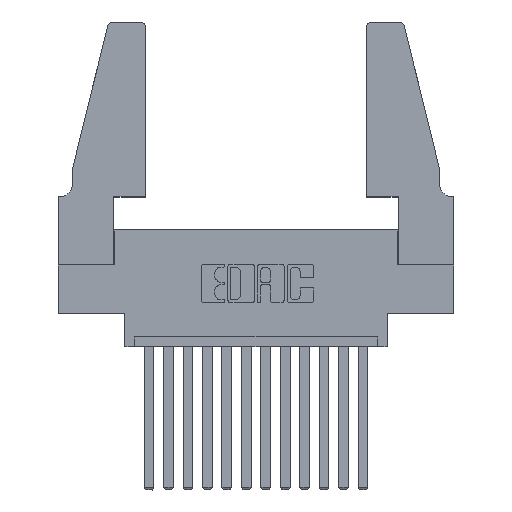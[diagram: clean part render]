
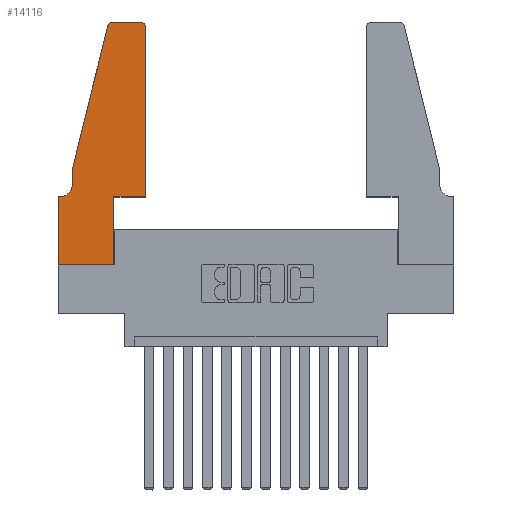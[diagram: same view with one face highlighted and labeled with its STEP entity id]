
A CAD part, top view. The second image highlights one B-rep face of the part: STEP entity #14116.
In plain terms, the highlighted planar face has unit normal (0, 0, 1).
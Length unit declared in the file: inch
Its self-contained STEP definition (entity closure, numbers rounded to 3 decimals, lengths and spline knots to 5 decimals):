
#272 = LINE ( 'NONE', #6849, #1726 ) ;
#416 = DIRECTION ( 'NONE',  ( 0., 0., 1. ) ) ;
#508 = EDGE_CURVE ( 'NONE', #1469, #7959, #272, .T. ) ;
#634 = DIRECTION ( 'NONE',  ( 0., 0., 1. ) ) ;
#906 = CARTESIAN_POINT ( 'NONE',  ( 0.0055, 0.35, 0.37 ) ) ;
#988 = LINE ( 'NONE', #8425, #2473 ) ;
#1020 = CARTESIAN_POINT ( 'NONE',  ( 0., 0.35, 0.37 ) ) ;
#1269 = DIRECTION ( 'NONE',  ( 0., -1., 0. ) ) ;
#1311 = CARTESIAN_POINT ( 'NONE',  ( 0.2865, 0.35, 0.37 ) ) ;
#1469 = VERTEX_POINT ( 'NONE', #1020 ) ;
#1584 = EDGE_CURVE ( 'NONE', #9518, #4187, #13650, .T. ) ;
#1589 = VERTEX_POINT ( 'NONE', #7172 ) ;
#1726 = VECTOR ( 'NONE', #7943, 39.37008 ) ;
#1871 = CARTESIAN_POINT ( 'NONE',  ( 0.4505, 0.35, 0.37 ) ) ;
#2280 = CARTESIAN_POINT ( 'NONE',  ( 0.4205, 1.25, 0.37 ) ) ;
#2445 = CARTESIAN_POINT ( 'NONE',  ( 0.284, 1.25, 0.37 ) ) ;
#2473 = VECTOR ( 'NONE', #1269, 39.37008 ) ;
#2568 = CARTESIAN_POINT ( 'NONE',  ( 0.4205, 1.22, 0.37 ) ) ;
#2576 = DIRECTION ( 'NONE',  ( 1., 0., 0. ) ) ;
#2619 = AXIS2_PLACEMENT_3D ( 'NONE', #14157, #12013, #7333 ) ;
#2770 = CARTESIAN_POINT ( 'NONE',  ( 0., 0., 0.37 ) ) ;
#3137 = EDGE_CURVE ( 'NONE', #7294, #11831, #12317, .T. ) ;
#3574 = EDGE_CURVE ( 'NONE', #11831, #5307, #11394, .T. ) ;
#3768 = VECTOR ( 'NONE', #7999, 39.37008 ) ;
#3900 = DIRECTION ( 'NONE',  ( 1., 0., 0. ) ) ;
#4038 = PLANE ( 'NONE',  #8104 ) ;
#4187 = VERTEX_POINT ( 'NONE', #906 ) ;
#4556 = EDGE_CURVE ( 'NONE', #4187, #1469, #12631, .T. ) ;
#4632 = FACE_OUTER_BOUND ( 'NONE', #12055, .T. ) ;
#4731 = VERTEX_POINT ( 'NONE', #11976 ) ;
#5307 = VERTEX_POINT ( 'NONE', #2445 ) ;
#5340 = DIRECTION ( 'NONE',  ( 0., 1., 0. ) ) ;
#5384 = CARTESIAN_POINT ( 'NONE',  ( 0.25487, 1.22718, 0.37 ) ) ;
#5847 = ORIENTED_EDGE ( 'NONE', *, *, #4556, .T. ) ;
#6104 = EDGE_CURVE ( 'NONE', #7457, #13045, #7702, .T. ) ;
#6130 = ORIENTED_EDGE ( 'NONE', *, *, #11282, .T. ) ;
#6164 = AXIS2_PLACEMENT_3D ( 'NONE', #6471, #416, #3900 ) ;
#6471 = CARTESIAN_POINT ( 'NONE',  ( 0.284, 1.22, 0.37 ) ) ;
#6482 = ORIENTED_EDGE ( 'NONE', *, *, #3137, .T. ) ;
#6849 = CARTESIAN_POINT ( 'NONE',  ( 0., 0., 0.37 ) ) ;
#6854 = LINE ( 'NONE', #9256, #14319 ) ;
#6967 = ORIENTED_EDGE ( 'NONE', *, *, #12311, .T. ) ;
#7172 = CARTESIAN_POINT ( 'NONE',  ( 0.2865, 0., 0.37 ) ) ;
#7294 = VERTEX_POINT ( 'NONE', #12242 ) ;
#7333 = DIRECTION ( 'NONE',  ( -1., 0., 0. ) ) ;
#7457 = VERTEX_POINT ( 'NONE', #1311 ) ;
#7500 = ORIENTED_EDGE ( 'NONE', *, *, #10553, .T. ) ;
#7589 = ORIENTED_EDGE ( 'NONE', *, *, #14219, .T. ) ;
#7674 = CARTESIAN_POINT ( 'NONE',  ( 0.0755, 0.42, 0.37 ) ) ;
#7702 = LINE ( 'NONE', #1871, #13156 ) ;
#7943 = DIRECTION ( 'NONE',  ( 0., -1., 0. ) ) ;
#7959 = VERTEX_POINT ( 'NONE', #9951 ) ;
#7999 = DIRECTION ( 'NONE',  ( 0., 1., 0. ) ) ;
#8104 = AXIS2_PLACEMENT_3D ( 'NONE', #8986, #634, #8930 ) ;
#8136 = EDGE_CURVE ( 'NONE', #5307, #8431, #10926, .T. ) ;
#8380 = CARTESIAN_POINT ( 'NONE',  ( 0.2605, 1.25, 0.37 ) ) ;
#8425 = CARTESIAN_POINT ( 'NONE',  ( 0.0755, 0.5, 0.37 ) ) ;
#8431 = VERTEX_POINT ( 'NONE', #5384 ) ;
#8471 = VECTOR ( 'NONE', #13333, 39.37008 ) ;
#8576 = CARTESIAN_POINT ( 'NONE',  ( 0.0755, 0.35, 0.37 ) ) ;
#8740 = DIRECTION ( 'NONE',  ( 1., 0., 0. ) ) ;
#8930 = DIRECTION ( 'NONE',  ( 1., 0., 0. ) ) ;
#8986 = CARTESIAN_POINT ( 'NONE',  ( 0., 0.35, 0.37 ) ) ;
#9180 = ORIENTED_EDGE ( 'NONE', *, *, #3574, .T. ) ;
#9256 = CARTESIAN_POINT ( 'NONE',  ( 0.0755, 0.5, 0.37 ) ) ;
#9468 = VECTOR ( 'NONE', #5340, 39.37008 ) ;
#9518 = VERTEX_POINT ( 'NONE', #7674 ) ;
#9621 = CARTESIAN_POINT ( 'NONE',  ( 0.4505, 0.35, 0.37 ) ) ;
#9951 = CARTESIAN_POINT ( 'NONE',  ( 0., 0., 0.37 ) ) ;
#10553 = EDGE_CURVE ( 'NONE', #1589, #7457, #12233, .T. ) ;
#10868 = DIRECTION ( 'NONE',  ( -1., 0., 0. ) ) ;
#10926 = CIRCLE ( 'NONE', #6164, 0.03 ) ;
#10998 = ORIENTED_EDGE ( 'NONE', *, *, #6104, .T. ) ;
#11282 = EDGE_CURVE ( 'NONE', #4731, #9518, #988, .T. ) ;
#11394 = LINE ( 'NONE', #8380, #12664 ) ;
#11831 = VERTEX_POINT ( 'NONE', #2280 ) ;
#11944 = LINE ( 'NONE', #2770, #12306 ) ;
#11976 = CARTESIAN_POINT ( 'NONE',  ( 0.0755, 0.5, 0.37 ) ) ;
#12013 = DIRECTION ( 'NONE',  ( 0., 0., -1. ) ) ;
#12055 = EDGE_LOOP ( 'NONE', ( #9180, #14656, #7589, #6130, #14744, #5847, #12659, #12304, #7500, #10998, #6967, #6482 ) ) ;
#12233 = LINE ( 'NONE', #13788, #3768 ) ;
#12242 = CARTESIAN_POINT ( 'NONE',  ( 0.4505, 1.22, 0.37 ) ) ;
#12304 = ORIENTED_EDGE ( 'NONE', *, *, #14585, .T. ) ;
#12306 = VECTOR ( 'NONE', #2576, 39.37008 ) ;
#12311 = EDGE_CURVE ( 'NONE', #13045, #7294, #13269, .T. ) ;
#12317 = CIRCLE ( 'NONE', #13244, 0.03 ) ;
#12348 = CARTESIAN_POINT ( 'NONE',  ( 0.4505, 0.35, 0.37 ) ) ;
#12631 = LINE ( 'NONE', #8576, #8471 ) ;
#12659 = ORIENTED_EDGE ( 'NONE', *, *, #508, .T. ) ;
#12664 = VECTOR ( 'NONE', #10868, 39.37008 ) ;
#12786 = DIRECTION ( 'NONE',  ( -0.239, -0.971, 0. ) ) ;
#13045 = VERTEX_POINT ( 'NONE', #9621 ) ;
#13156 = VECTOR ( 'NONE', #13725, 39.37008 ) ;
#13244 = AXIS2_PLACEMENT_3D ( 'NONE', #2568, #13393, #8740 ) ;
#13269 = LINE ( 'NONE', #12348, #9468 ) ;
#13333 = DIRECTION ( 'NONE',  ( -1., 0., 0. ) ) ;
#13393 = DIRECTION ( 'NONE',  ( 0., 0., 1. ) ) ;
#13650 = CIRCLE ( 'NONE', #2619, 0.07 ) ;
#13725 = DIRECTION ( 'NONE',  ( 1., 0., 0. ) ) ;
#13788 = CARTESIAN_POINT ( 'NONE',  ( 0.2865, 0.35, 0.37 ) ) ;
#14116 = ADVANCED_FACE ( 'NONE', ( #4632 ), #4038, .T. ) ;
#14157 = CARTESIAN_POINT ( 'NONE',  ( 0.0055, 0.42, 0.37 ) ) ;
#14219 = EDGE_CURVE ( 'NONE', #8431, #4731, #6854, .T. ) ;
#14319 = VECTOR ( 'NONE', #12786, 39.37008 ) ;
#14585 = EDGE_CURVE ( 'NONE', #7959, #1589, #11944, .T. ) ;
#14656 = ORIENTED_EDGE ( 'NONE', *, *, #8136, .T. ) ;
#14744 = ORIENTED_EDGE ( 'NONE', *, *, #1584, .T. ) ;
